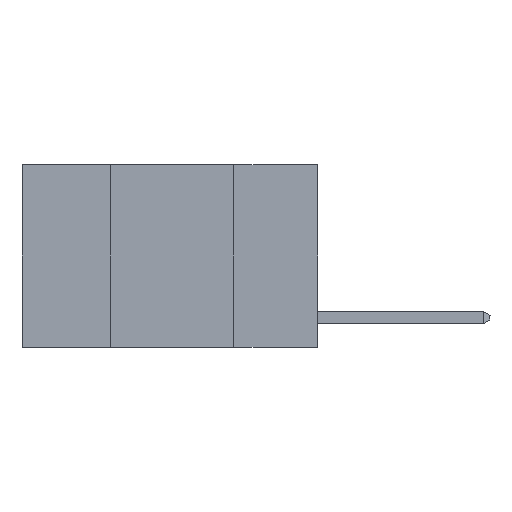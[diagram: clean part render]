
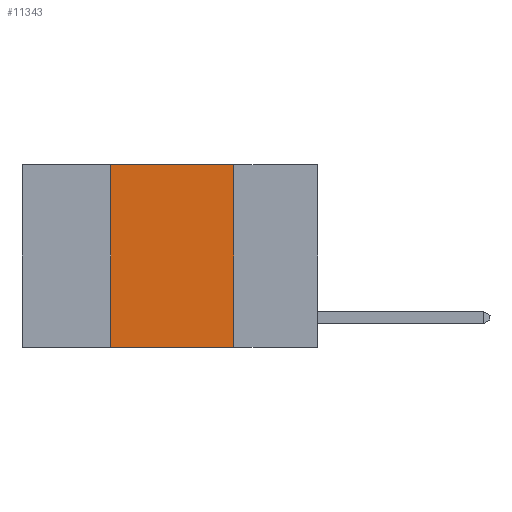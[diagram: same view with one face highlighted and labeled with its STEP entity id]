
A CAD part, left-side view. The second image highlights one B-rep face of the part: STEP entity #11343.
In plain terms, the highlighted planar face has unit normal (-1, 0, 0).
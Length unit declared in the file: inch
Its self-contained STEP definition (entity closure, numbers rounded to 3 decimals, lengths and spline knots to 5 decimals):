
#707 = CARTESIAN_POINT ( 'NONE',  ( 0., 0.17, 0. ) ) ;
#850 = VERTEX_POINT ( 'NONE', #707 ) ;
#1141 = EDGE_CURVE ( 'NONE', #11317, #1790, #14236, .T. ) ;
#1200 = CARTESIAN_POINT ( 'NONE',  ( 0., 0.17, -0.37 ) ) ;
#1327 = CARTESIAN_POINT ( 'NONE',  ( 0., 0.42, 0. ) ) ;
#1790 = VERTEX_POINT ( 'NONE', #12993 ) ;
#2655 = LINE ( 'NONE', #14376, #15491 ) ;
#4555 = PLANE ( 'NONE',  #9380 ) ;
#4614 = EDGE_CURVE ( 'NONE', #850, #13725, #10294, .T. ) ;
#4894 = CARTESIAN_POINT ( 'NONE',  ( 0., 0.17, 0. ) ) ;
#5866 = DIRECTION ( 'NONE',  ( 1., 0., 0. ) ) ;
#5875 = DIRECTION ( 'NONE',  ( 0., -1., 0. ) ) ;
#5885 = VECTOR ( 'NONE', #7608, 39.37008 ) ;
#6655 = VECTOR ( 'NONE', #8717, 39.37008 ) ;
#6840 = DIRECTION ( 'NONE',  ( 0., 0., 1. ) ) ;
#7608 = DIRECTION ( 'NONE',  ( 0., -1., 0. ) ) ;
#7815 = VECTOR ( 'NONE', #6840, 39.37008 ) ;
#8717 = DIRECTION ( 'NONE',  ( 0., 0., -1. ) ) ;
#9380 = AXIS2_PLACEMENT_3D ( 'NONE', #13193, #5866, #14422 ) ;
#9458 = ORIENTED_EDGE ( 'NONE', *, *, #11573, .T. ) ;
#10292 = EDGE_CURVE ( 'NONE', #1790, #850, #2655, .T. ) ;
#10294 = LINE ( 'NONE', #4894, #6655 ) ;
#11317 = VERTEX_POINT ( 'NONE', #14369 ) ;
#11343 = ADVANCED_FACE ( 'NONE', ( #15474 ), #4555, .F. ) ;
#11573 = EDGE_CURVE ( 'NONE', #11317, #13725, #12402, .T. ) ;
#12283 = ORIENTED_EDGE ( 'NONE', *, *, #10292, .F. ) ;
#12402 = LINE ( 'NONE', #14856, #5885 ) ;
#12714 = EDGE_LOOP ( 'NONE', ( #15162, #12283, #15540, #9458 ) ) ;
#12993 = CARTESIAN_POINT ( 'NONE',  ( 0., 0.42, 0. ) ) ;
#13193 = CARTESIAN_POINT ( 'NONE',  ( 0., 0.6, 0. ) ) ;
#13725 = VERTEX_POINT ( 'NONE', #1200 ) ;
#14236 = LINE ( 'NONE', #1327, #7815 ) ;
#14369 = CARTESIAN_POINT ( 'NONE',  ( 0., 0.42, -0.37 ) ) ;
#14376 = CARTESIAN_POINT ( 'NONE',  ( 0., 0.6, 0. ) ) ;
#14422 = DIRECTION ( 'NONE',  ( 0., 0., -1. ) ) ;
#14856 = CARTESIAN_POINT ( 'NONE',  ( 0., 0.6, -0.37 ) ) ;
#15162 = ORIENTED_EDGE ( 'NONE', *, *, #4614, .F. ) ;
#15474 = FACE_OUTER_BOUND ( 'NONE', #12714, .T. ) ;
#15491 = VECTOR ( 'NONE', #5875, 39.37008 ) ;
#15540 = ORIENTED_EDGE ( 'NONE', *, *, #1141, .F. ) ;
